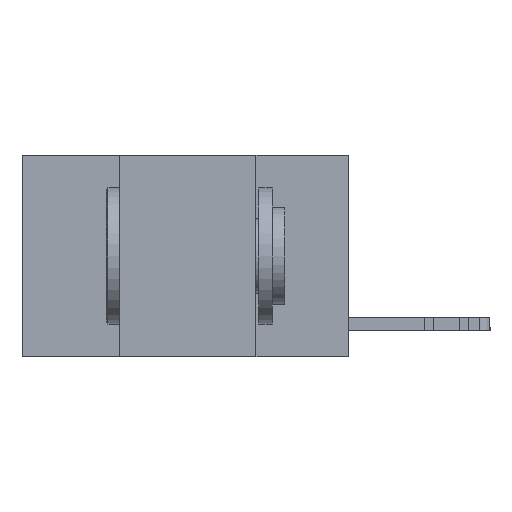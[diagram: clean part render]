
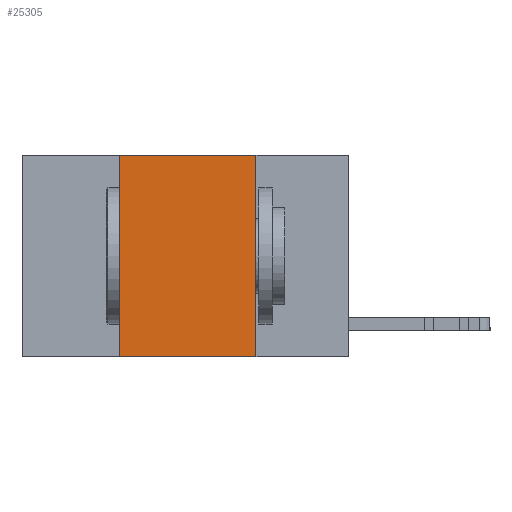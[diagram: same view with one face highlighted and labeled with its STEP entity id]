
A CAD part, left-side view. The second image highlights one B-rep face of the part: STEP entity #25305.
In plain terms, the highlighted planar face has unit normal (-1, 0, 0).
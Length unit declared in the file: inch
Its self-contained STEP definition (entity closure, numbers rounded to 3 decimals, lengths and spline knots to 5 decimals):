
#1125 = CARTESIAN_POINT ( 'NONE',  ( 0., 0.6, 0. ) ) ;
#1959 = LINE ( 'NONE', #9088, #12772 ) ;
#2238 = CARTESIAN_POINT ( 'NONE',  ( 0., 0.17, 0. ) ) ;
#4308 = VECTOR ( 'NONE', #8712, 39.37008 ) ;
#5666 = PLANE ( 'NONE',  #17680 ) ;
#6896 = EDGE_CURVE ( 'NONE', #22761, #28014, #1959, .T. ) ;
#7853 = LINE ( 'NONE', #16701, #4308 ) ;
#8125 = VECTOR ( 'NONE', #24025, 39.37008 ) ;
#8175 = EDGE_CURVE ( 'NONE', #12175, #19775, #13278, .T. ) ;
#8712 = DIRECTION ( 'NONE',  ( 0., -1., 0. ) ) ;
#9088 = CARTESIAN_POINT ( 'NONE',  ( 0., 0.17, 0. ) ) ;
#9662 = DIRECTION ( 'NONE',  ( 0., -1., 0. ) ) ;
#10979 = CARTESIAN_POINT ( 'NONE',  ( 0., 0.42, 0. ) ) ;
#12175 = VERTEX_POINT ( 'NONE', #22758 ) ;
#12637 = CARTESIAN_POINT ( 'NONE',  ( 0., 0.17, -0.37 ) ) ;
#12772 = VECTOR ( 'NONE', #15324, 39.37008 ) ;
#13278 = LINE ( 'NONE', #10979, #8125 ) ;
#14639 = ORIENTED_EDGE ( 'NONE', *, *, #6896, .F. ) ;
#15324 = DIRECTION ( 'NONE',  ( 0., 0., -1. ) ) ;
#16480 = LINE ( 'NONE', #27221, #27904 ) ;
#16701 = CARTESIAN_POINT ( 'NONE',  ( 0., 0.6, 0. ) ) ;
#16787 = ORIENTED_EDGE ( 'NONE', *, *, #25530, .T. ) ;
#17680 = AXIS2_PLACEMENT_3D ( 'NONE', #1125, #19044, #19192 ) ;
#19044 = DIRECTION ( 'NONE',  ( 1., 0., 0. ) ) ;
#19192 = DIRECTION ( 'NONE',  ( 0., 0., -1. ) ) ;
#19775 = VERTEX_POINT ( 'NONE', #26229 ) ;
#21267 = ORIENTED_EDGE ( 'NONE', *, *, #8175, .F. ) ;
#22758 = CARTESIAN_POINT ( 'NONE',  ( 0., 0.42, -0.37 ) ) ;
#22761 = VERTEX_POINT ( 'NONE', #2238 ) ;
#24025 = DIRECTION ( 'NONE',  ( 0., 0., 1. ) ) ;
#25305 = ADVANCED_FACE ( 'NONE', ( #28187 ), #5666, .F. ) ;
#25530 = EDGE_CURVE ( 'NONE', #12175, #28014, #16480, .T. ) ;
#26229 = CARTESIAN_POINT ( 'NONE',  ( 0., 0.42, 0. ) ) ;
#26265 = ORIENTED_EDGE ( 'NONE', *, *, #26762, .F. ) ;
#26762 = EDGE_CURVE ( 'NONE', #19775, #22761, #7853, .T. ) ;
#27221 = CARTESIAN_POINT ( 'NONE',  ( 0., 0.6, -0.37 ) ) ;
#27226 = EDGE_LOOP ( 'NONE', ( #14639, #26265, #21267, #16787 ) ) ;
#27904 = VECTOR ( 'NONE', #9662, 39.37008 ) ;
#28014 = VERTEX_POINT ( 'NONE', #12637 ) ;
#28187 = FACE_OUTER_BOUND ( 'NONE', #27226, .T. ) ;
